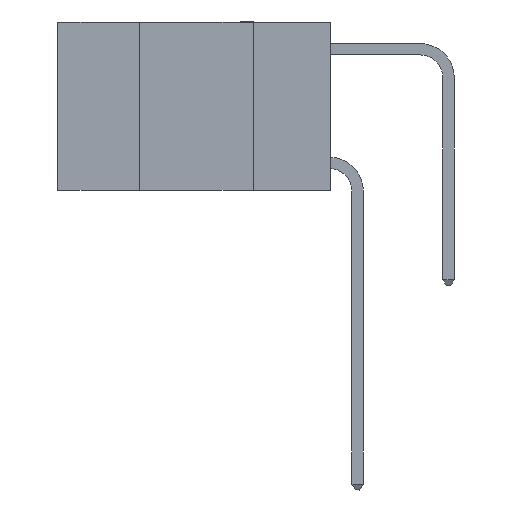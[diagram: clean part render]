
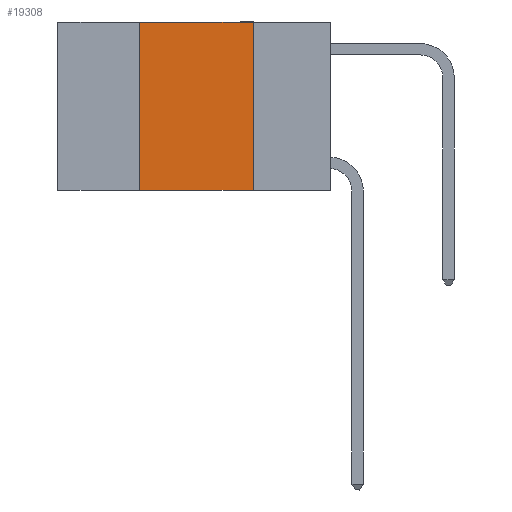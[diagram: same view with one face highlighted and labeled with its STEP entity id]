
A CAD part, left-side view. The second image highlights one B-rep face of the part: STEP entity #19308.
In plain terms, the highlighted planar face has unit normal (-1, 0, 0).
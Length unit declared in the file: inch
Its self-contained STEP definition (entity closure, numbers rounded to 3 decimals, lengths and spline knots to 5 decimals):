
#353 = VECTOR ( 'NONE', #8857, 39.37008 ) ;
#1566 = CARTESIAN_POINT ( 'NONE',  ( 0., 0.6, 0. ) ) ;
#2003 = ORIENTED_EDGE ( 'NONE', *, *, #8715, .F. ) ;
#3145 = ORIENTED_EDGE ( 'NONE', *, *, #10323, .F. ) ;
#3949 = CARTESIAN_POINT ( 'NONE',  ( 0., 0.17, -0.37 ) ) ;
#4485 = EDGE_CURVE ( 'NONE', #9152, #16484, #16636, .T. ) ;
#5307 = DIRECTION ( 'NONE',  ( 1., 0., 0. ) ) ;
#5390 = VECTOR ( 'NONE', #12872, 39.37008 ) ;
#5702 = CARTESIAN_POINT ( 'NONE',  ( 0., 0.42, 0. ) ) ;
#6539 = ORIENTED_EDGE ( 'NONE', *, *, #4485, .F. ) ;
#7407 = CARTESIAN_POINT ( 'NONE',  ( 0., 0.17, 0. ) ) ;
#7725 = EDGE_LOOP ( 'NONE', ( #2003, #6539, #3145, #19995 ) ) ;
#7812 = CARTESIAN_POINT ( 'NONE',  ( 0., 0.42, -0.37 ) ) ;
#8056 = VECTOR ( 'NONE', #10695, 39.37008 ) ;
#8272 = LINE ( 'NONE', #20255, #5390 ) ;
#8715 = EDGE_CURVE ( 'NONE', #16484, #11305, #8272, .T. ) ;
#8736 = CARTESIAN_POINT ( 'NONE',  ( 0., 0.6, -0.37 ) ) ;
#8857 = DIRECTION ( 'NONE',  ( 0., -1., 0. ) ) ;
#9152 = VERTEX_POINT ( 'NONE', #5702 ) ;
#9500 = DIRECTION ( 'NONE',  ( 0., 0., 1. ) ) ;
#10323 = EDGE_CURVE ( 'NONE', #15924, #9152, #20684, .T. ) ;
#10695 = DIRECTION ( 'NONE',  ( 0., -1., 0. ) ) ;
#11305 = VERTEX_POINT ( 'NONE', #3949 ) ;
#12475 = PLANE ( 'NONE',  #21992 ) ;
#12872 = DIRECTION ( 'NONE',  ( 0., 0., -1. ) ) ;
#14454 = EDGE_CURVE ( 'NONE', #15924, #11305, #14746, .T. ) ;
#14746 = LINE ( 'NONE', #8736, #8056 ) ;
#15924 = VERTEX_POINT ( 'NONE', #7812 ) ;
#16484 = VERTEX_POINT ( 'NONE', #7407 ) ;
#16636 = LINE ( 'NONE', #21501, #353 ) ;
#19033 = VECTOR ( 'NONE', #9500, 39.37008 ) ;
#19308 = ADVANCED_FACE ( 'NONE', ( #19732 ), #12475, .F. ) ;
#19732 = FACE_OUTER_BOUND ( 'NONE', #7725, .T. ) ;
#19995 = ORIENTED_EDGE ( 'NONE', *, *, #14454, .T. ) ;
#20155 = CARTESIAN_POINT ( 'NONE',  ( 0., 0.42, 0. ) ) ;
#20255 = CARTESIAN_POINT ( 'NONE',  ( 0., 0.17, 0. ) ) ;
#20684 = LINE ( 'NONE', #20155, #19033 ) ;
#21471 = DIRECTION ( 'NONE',  ( 0., 0., -1. ) ) ;
#21501 = CARTESIAN_POINT ( 'NONE',  ( 0., 0.6, 0. ) ) ;
#21992 = AXIS2_PLACEMENT_3D ( 'NONE', #1566, #5307, #21471 ) ;
